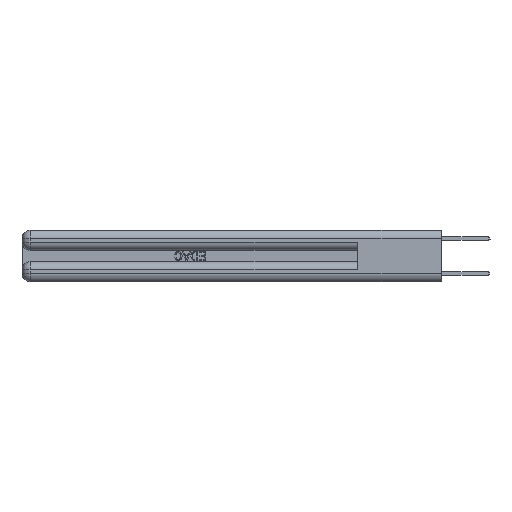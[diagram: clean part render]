
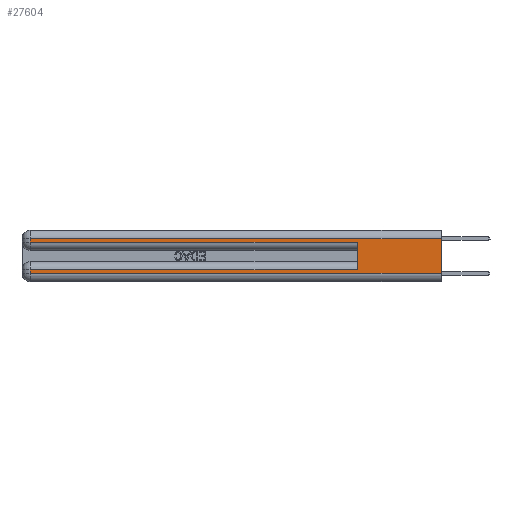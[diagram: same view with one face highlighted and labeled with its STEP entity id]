
A CAD part, left-side view. The second image highlights one B-rep face of the part: STEP entity #27604.
In plain terms, the highlighted planar face has unit normal (-1, 0, 0).
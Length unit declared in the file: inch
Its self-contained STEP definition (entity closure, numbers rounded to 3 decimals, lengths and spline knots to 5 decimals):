
#82 = CARTESIAN_POINT ( 'NONE',  ( 0., 0., 0.06 ) ) ;
#270 = PLANE ( 'NONE',  #4056 ) ;
#540 = CARTESIAN_POINT ( 'NONE',  ( 0., 0., 0.31 ) ) ;
#567 = VERTEX_POINT ( 'NONE', #540 ) ;
#1032 = VECTOR ( 'NONE', #22879, 39.37008 ) ;
#2263 = VERTEX_POINT ( 'NONE', #9227 ) ;
#2490 = CARTESIAN_POINT ( 'NONE',  ( 0., 0., 0.085 ) ) ;
#2492 = ORIENTED_EDGE ( 'NONE', *, *, #12391, .T. ) ;
#2814 = LINE ( 'NONE', #2490, #16323 ) ;
#2957 = CARTESIAN_POINT ( 'NONE',  ( 0., 2.94, 0.06 ) ) ;
#3020 = VERTEX_POINT ( 'NONE', #21802 ) ;
#3099 = LINE ( 'NONE', #20679, #4928 ) ;
#4056 = AXIS2_PLACEMENT_3D ( 'NONE', #24204, #17077, #24315 ) ;
#4928 = VECTOR ( 'NONE', #25617, 39.37008 ) ;
#4994 = CARTESIAN_POINT ( 'NONE',  ( 0., 0.6, 0.145 ) ) ;
#5126 = VERTEX_POINT ( 'NONE', #2957 ) ;
#5396 = EDGE_CURVE ( 'NONE', #567, #3020, #14984, .T. ) ;
#5728 = LINE ( 'NONE', #14046, #12506 ) ;
#6459 = VERTEX_POINT ( 'NONE', #20039 ) ;
#6607 = DIRECTION ( 'NONE',  ( 0., 0., -1. ) ) ;
#7723 = CARTESIAN_POINT ( 'NONE',  ( 0., 0., 0.31 ) ) ;
#7775 = CARTESIAN_POINT ( 'NONE',  ( 0., 2.94, 0.37 ) ) ;
#8004 = ORIENTED_EDGE ( 'NONE', *, *, #27938, .T. ) ;
#8262 = ORIENTED_EDGE ( 'NONE', *, *, #27685, .T. ) ;
#8762 = EDGE_CURVE ( 'NONE', #9867, #2263, #24294, .T. ) ;
#9227 = CARTESIAN_POINT ( 'NONE',  ( 0., 0.6, 0.285 ) ) ;
#9626 = ORIENTED_EDGE ( 'NONE', *, *, #13281, .T. ) ;
#9867 = VERTEX_POINT ( 'NONE', #13226 ) ;
#9935 = ORIENTED_EDGE ( 'NONE', *, *, #8762, .T. ) ;
#10127 = VECTOR ( 'NONE', #22189, 39.37008 ) ;
#10369 = DIRECTION ( 'NONE',  ( 0., 1., 0. ) ) ;
#11665 = LINE ( 'NONE', #7775, #12049 ) ;
#12049 = VECTOR ( 'NONE', #26657, 39.37008 ) ;
#12391 = EDGE_CURVE ( 'NONE', #6459, #5126, #3099, .T. ) ;
#12506 = VECTOR ( 'NONE', #6607, 39.37008 ) ;
#12833 = CARTESIAN_POINT ( 'NONE',  ( 0., 0.6, 0.085 ) ) ;
#13132 = VERTEX_POINT ( 'NONE', #82 ) ;
#13226 = CARTESIAN_POINT ( 'NONE',  ( 0., 2.94, 0.285 ) ) ;
#13281 = EDGE_CURVE ( 'NONE', #3020, #9867, #11665, .T. ) ;
#13342 = LINE ( 'NONE', #4994, #21182 ) ;
#14046 = CARTESIAN_POINT ( 'NONE',  ( 0., 0., 0.37 ) ) ;
#14406 = ORIENTED_EDGE ( 'NONE', *, *, #23735, .F. ) ;
#14469 = FACE_OUTER_BOUND ( 'NONE', #24999, .T. ) ;
#14984 = LINE ( 'NONE', #7723, #10127 ) ;
#15847 = CARTESIAN_POINT ( 'NONE',  ( 0., 0., 0.285 ) ) ;
#16323 = VECTOR ( 'NONE', #10369, 39.37008 ) ;
#17077 = DIRECTION ( 'NONE',  ( 1., 0., 0. ) ) ;
#18958 = VECTOR ( 'NONE', #25141, 39.37008 ) ;
#20039 = CARTESIAN_POINT ( 'NONE',  ( 0., 2.94, 0.085 ) ) ;
#20679 = CARTESIAN_POINT ( 'NONE',  ( 0., 2.94, 0.37 ) ) ;
#21182 = VECTOR ( 'NONE', #29156, 39.37008 ) ;
#21383 = ORIENTED_EDGE ( 'NONE', *, *, #27618, .F. ) ;
#21802 = CARTESIAN_POINT ( 'NONE',  ( 0., 2.94, 0.31 ) ) ;
#22189 = DIRECTION ( 'NONE',  ( 0., 1., 0. ) ) ;
#22726 = CARTESIAN_POINT ( 'NONE',  ( 0., 0., 0.06 ) ) ;
#22879 = DIRECTION ( 'NONE',  ( 0., -1., 0. ) ) ;
#23394 = ORIENTED_EDGE ( 'NONE', *, *, #5396, .T. ) ;
#23735 = EDGE_CURVE ( 'NONE', #567, #13132, #5728, .T. ) ;
#24204 = CARTESIAN_POINT ( 'NONE',  ( 0., 0., 0.37 ) ) ;
#24294 = LINE ( 'NONE', #15847, #1032 ) ;
#24315 = DIRECTION ( 'NONE',  ( 0., 0., -1. ) ) ;
#24999 = EDGE_LOOP ( 'NONE', ( #14406, #23394, #9626, #9935, #21383, #8262, #2492, #8004 ) ) ;
#25141 = DIRECTION ( 'NONE',  ( 0., -1., 0. ) ) ;
#25617 = DIRECTION ( 'NONE',  ( 0., 0., -1. ) ) ;
#25726 = LINE ( 'NONE', #22726, #18958 ) ;
#26657 = DIRECTION ( 'NONE',  ( 0., 0., -1. ) ) ;
#27604 = ADVANCED_FACE ( 'NONE', ( #14469 ), #270, .F. ) ;
#27618 = EDGE_CURVE ( 'NONE', #30808, #2263, #13342, .T. ) ;
#27685 = EDGE_CURVE ( 'NONE', #30808, #6459, #2814, .T. ) ;
#27938 = EDGE_CURVE ( 'NONE', #5126, #13132, #25726, .T. ) ;
#29156 = DIRECTION ( 'NONE',  ( 0., 0., 1. ) ) ;
#30808 = VERTEX_POINT ( 'NONE', #12833 ) ;
